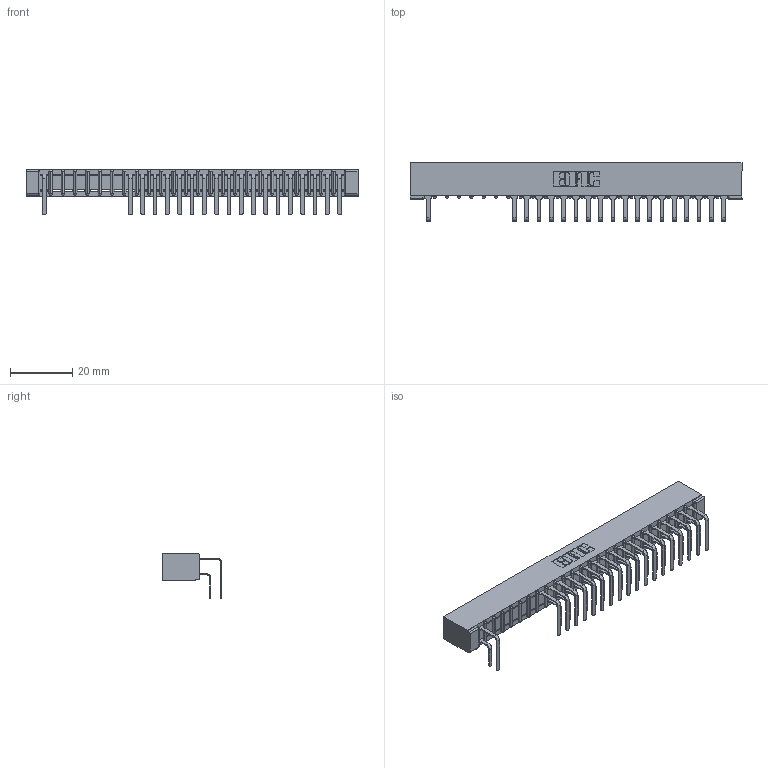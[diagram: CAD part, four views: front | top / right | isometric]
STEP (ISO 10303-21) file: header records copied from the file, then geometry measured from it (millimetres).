
FILE_DESCRIPTION (( 'STEP AP203' ), '1' );
FILE_NAME ('307-025-558-101.STEP', '2018-08-04T08:01:40', ( '' ), ( '' ), 'SwSTEP 2.0', 'SolidWorks 2016', '' );
FILE_SCHEMA (( 'CONFIG_CONTROL_DESIGN' ));
Length unit declared in the file: inch
Products named in the file (4): 307 Part_No Mounting Lugs; 307-290-001_558 559 - 1 (Single); 307-290-001_558 - 2 (Single); 307-025-558-101
Assembly tree (38 placements, depth 2):
  307-025-558-101
    307 Part_No Mounting Lugs
    307-290-001_558 559 - 1 (Single)  x18
    307-290-001_558 - 2 (Single)  x19
Bounding box: 106.93 x 18.96 x 14.81 mm (x, y, z)
Volume: 7224.8 mm3; surface area: 13327.2 mm2
Topology: 38 solids, 38 shells, 2116 faces, 5969 edges, 3858 vertices
Faces by surface type: plane 1365, cylinder 699, sphere 52
Entity records: 25081 total; most frequent: CARTESIAN_POINT 4162, ORIENTED_EDGE 4134, DIRECTION 4069, EDGE_CURVE 2067, VECTOR 1579, LINE 1579, VERTEX_POINT 1338, AXIS2_PLACEMENT_3D 1245
